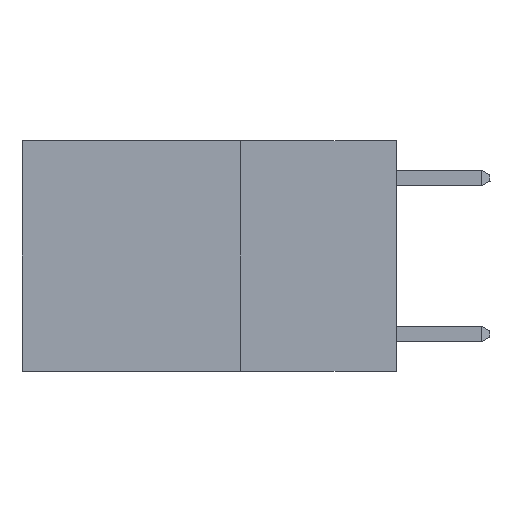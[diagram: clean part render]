
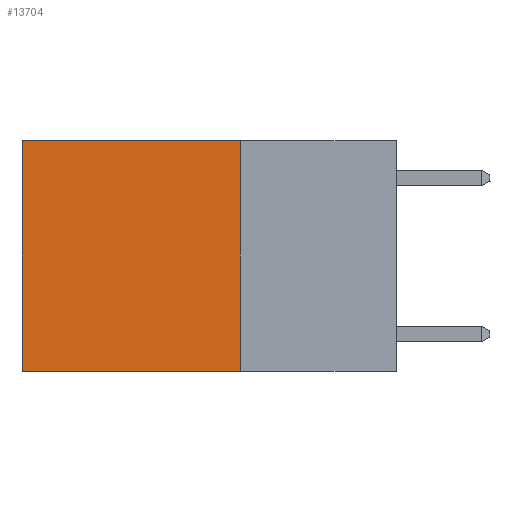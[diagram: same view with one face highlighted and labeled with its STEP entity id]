
A CAD part, left-side view. The second image highlights one B-rep face of the part: STEP entity #13704.
In plain terms, the highlighted planar face has unit normal (-1, 0, 0).
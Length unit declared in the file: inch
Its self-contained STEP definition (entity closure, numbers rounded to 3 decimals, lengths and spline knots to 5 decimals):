
#547 = PLANE ( 'NONE',  #9362 ) ;
#754 = ORIENTED_EDGE ( 'NONE', *, *, #933, .F. ) ;
#858 = ORIENTED_EDGE ( 'NONE', *, *, #3425, .T. ) ;
#933 = EDGE_CURVE ( 'NONE', #15432, #16152, #4793, .T. ) ;
#1860 = DIRECTION ( 'NONE',  ( 0., 0., -1. ) ) ;
#2142 = CARTESIAN_POINT ( 'NONE',  ( 0.2625, 0.25, -0.37 ) ) ;
#2342 = LINE ( 'NONE', #14771, #5412 ) ;
#2378 = LINE ( 'NONE', #10525, #12388 ) ;
#2745 = FACE_OUTER_BOUND ( 'NONE', #7935, .T. ) ;
#3177 = CARTESIAN_POINT ( 'NONE',  ( 0.2625, 0.25, 0. ) ) ;
#3425 = EDGE_CURVE ( 'NONE', #7144, #16152, #2378, .T. ) ;
#4793 = LINE ( 'NONE', #10981, #14682 ) ;
#5412 = VECTOR ( 'NONE', #5776, 39.37008 ) ;
#5580 = VECTOR ( 'NONE', #12359, 39.37008 ) ;
#5754 = CARTESIAN_POINT ( 'NONE',  ( 0.2625, 0.25, 0. ) ) ;
#5776 = DIRECTION ( 'NONE',  ( 0., 1., 0. ) ) ;
#6011 = EDGE_CURVE ( 'NONE', #12469, #15432, #9096, .T. ) ;
#6518 = ORIENTED_EDGE ( 'NONE', *, *, #15245, .T. ) ;
#7019 = DIRECTION ( 'NONE',  ( 0., 1., 0. ) ) ;
#7026 = CARTESIAN_POINT ( 'NONE',  ( 0.2625, 0.25, 0. ) ) ;
#7144 = VERTEX_POINT ( 'NONE', #13479 ) ;
#7935 = EDGE_LOOP ( 'NONE', ( #858, #754, #8600, #6518 ) ) ;
#8600 = ORIENTED_EDGE ( 'NONE', *, *, #6011, .F. ) ;
#9096 = LINE ( 'NONE', #3177, #5580 ) ;
#9362 = AXIS2_PLACEMENT_3D ( 'NONE', #7026, #9712, #1860 ) ;
#9712 = DIRECTION ( 'NONE',  ( 1., 0., 0. ) ) ;
#10525 = CARTESIAN_POINT ( 'NONE',  ( 0.2625, 0.6, 0. ) ) ;
#10579 = DIRECTION ( 'NONE',  ( 0., 0., -1. ) ) ;
#10981 = CARTESIAN_POINT ( 'NONE',  ( 0.2625, 0.25, -0.37 ) ) ;
#12359 = DIRECTION ( 'NONE',  ( 0., 0., -1. ) ) ;
#12388 = VECTOR ( 'NONE', #10579, 39.37008 ) ;
#12469 = VERTEX_POINT ( 'NONE', #5754 ) ;
#13479 = CARTESIAN_POINT ( 'NONE',  ( 0.2625, 0.6, 0. ) ) ;
#13704 = ADVANCED_FACE ( 'NONE', ( #2745 ), #547, .F. ) ;
#14682 = VECTOR ( 'NONE', #7019, 39.37008 ) ;
#14771 = CARTESIAN_POINT ( 'NONE',  ( 0.2625, 0.25, 0. ) ) ;
#15189 = CARTESIAN_POINT ( 'NONE',  ( 0.2625, 0.6, -0.37 ) ) ;
#15245 = EDGE_CURVE ( 'NONE', #12469, #7144, #2342, .T. ) ;
#15432 = VERTEX_POINT ( 'NONE', #2142 ) ;
#16152 = VERTEX_POINT ( 'NONE', #15189 ) ;
